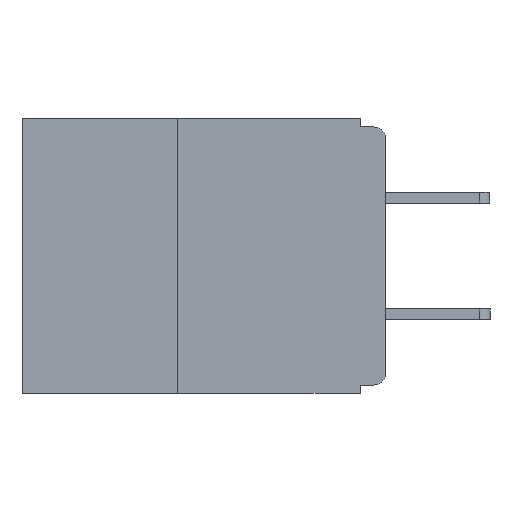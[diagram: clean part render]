
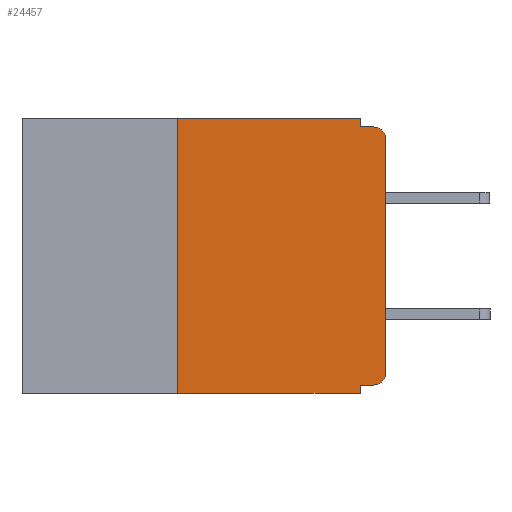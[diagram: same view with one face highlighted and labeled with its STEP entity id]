
A CAD part, left-side view. The second image highlights one B-rep face of the part: STEP entity #24457.
In plain terms, the highlighted planar face has unit normal (-1, 0, 0).
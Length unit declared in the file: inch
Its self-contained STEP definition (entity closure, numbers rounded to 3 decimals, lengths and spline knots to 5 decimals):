
#37 = VERTEX_POINT ( 'NONE', #17384 ) ;
#172 = LINE ( 'NONE', #26033, #16904 ) ;
#1233 = CIRCLE ( 'NONE', #4353, 0.015 ) ;
#1539 = LINE ( 'NONE', #8514, #12045 ) ;
#1706 = VERTEX_POINT ( 'NONE', #14903 ) ;
#2119 = VECTOR ( 'NONE', #4753, 39.37008 ) ;
#3079 = CARTESIAN_POINT ( 'NONE',  ( 0., 0.437, -0.33 ) ) ;
#3104 = DIRECTION ( 'NONE',  ( 0., -1., 0. ) ) ;
#3192 = EDGE_CURVE ( 'NONE', #7792, #24242, #1233, .T. ) ;
#3347 = CARTESIAN_POINT ( 'NONE',  ( 0., 0., -0.025 ) ) ;
#3579 = DIRECTION ( 'NONE',  ( 0., 0., -1. ) ) ;
#4067 = EDGE_CURVE ( 'NONE', #7661, #21349, #1539, .T. ) ;
#4260 = EDGE_LOOP ( 'NONE', ( #22981, #23502, #23554, #24234, #24512, #24639, #25040, #25345, #25352, #25629 ) ) ;
#4353 = AXIS2_PLACEMENT_3D ( 'NONE', #6481, #6469, #6438 ) ;
#4753 = DIRECTION ( 'NONE',  ( 0., 0., 1. ) ) ;
#4786 = CARTESIAN_POINT ( 'NONE',  ( 0., 0., 0. ) ) ;
#5506 = EDGE_CURVE ( 'NONE', #21349, #19329, #11683, .T. ) ;
#5776 = EDGE_CURVE ( 'NONE', #19329, #15866, #26083, .T. ) ;
#6105 = EDGE_CURVE ( 'NONE', #24242, #11061, #12623, .T. ) ;
#6438 = DIRECTION ( 'NONE',  ( 0., 0., -1. ) ) ;
#6469 = DIRECTION ( 'NONE',  ( -1., 0., 0. ) ) ;
#6481 = CARTESIAN_POINT ( 'NONE',  ( 0., 0.015, -0.305 ) ) ;
#7461 = PLANE ( 'NONE',  #7885 ) ;
#7475 = EDGE_CURVE ( 'NONE', #7792, #17585, #16513, .T. ) ;
#7661 = VERTEX_POINT ( 'NONE', #21266 ) ;
#7792 = VERTEX_POINT ( 'NONE', #18733 ) ;
#7885 = AXIS2_PLACEMENT_3D ( 'NONE', #9550, #11694, #26331 ) ;
#7938 = CARTESIAN_POINT ( 'NONE',  ( 0., 0.015, -0.025 ) ) ;
#8514 = CARTESIAN_POINT ( 'NONE',  ( 0., 0.25, -0.33 ) ) ;
#8648 = CARTESIAN_POINT ( 'NONE',  ( 0., 0., -0.305 ) ) ;
#8722 = CARTESIAN_POINT ( 'NONE',  ( 0., 0.031, -0.32 ) ) ;
#8989 = EDGE_CURVE ( 'NONE', #7661, #37, #23648, .T. ) ;
#9550 = CARTESIAN_POINT ( 'NONE',  ( 0., 0.437, 0. ) ) ;
#10058 = DIRECTION ( 'NONE',  ( 0., 0., -1. ) ) ;
#10143 = FACE_OUTER_BOUND ( 'NONE', #4260, .T. ) ;
#11061 = VERTEX_POINT ( 'NONE', #3347 ) ;
#11683 = LINE ( 'NONE', #17217, #16585 ) ;
#11694 = DIRECTION ( 'NONE',  ( 1., 0., 0. ) ) ;
#11939 = DIRECTION ( 'NONE',  ( 0., 0., -1. ) ) ;
#12045 = VECTOR ( 'NONE', #15084, 39.37008 ) ;
#12138 = CARTESIAN_POINT ( 'NONE',  ( 0., 0.031, 0. ) ) ;
#12623 = LINE ( 'NONE', #4786, #2119 ) ;
#13485 = DIRECTION ( 'NONE',  ( 0., -1., 0. ) ) ;
#13922 = EDGE_CURVE ( 'NONE', #17585, #37, #25687, .T. ) ;
#14903 = CARTESIAN_POINT ( 'NONE',  ( 0., 0.015, -0.01 ) ) ;
#15084 = DIRECTION ( 'NONE',  ( 0., 0., 1. ) ) ;
#15177 = VECTOR ( 'NONE', #3579, 39.37008 ) ;
#15866 = VERTEX_POINT ( 'NONE', #17449 ) ;
#16513 = LINE ( 'NONE', #23164, #26974 ) ;
#16585 = VECTOR ( 'NONE', #17040, 39.37008 ) ;
#16904 = VECTOR ( 'NONE', #13485, 39.37008 ) ;
#17040 = DIRECTION ( 'NONE',  ( 0., -1., 0. ) ) ;
#17217 = CARTESIAN_POINT ( 'NONE',  ( 0., 0.437, 0. ) ) ;
#17384 = CARTESIAN_POINT ( 'NONE',  ( 0., 0.031, -0.33 ) ) ;
#17449 = CARTESIAN_POINT ( 'NONE',  ( 0., 0.031, -0.01 ) ) ;
#17585 = VERTEX_POINT ( 'NONE', #8722 ) ;
#18733 = CARTESIAN_POINT ( 'NONE',  ( 0., 0.015, -0.32 ) ) ;
#18740 = VECTOR ( 'NONE', #3104, 39.37008 ) ;
#19329 = VERTEX_POINT ( 'NONE', #22797 ) ;
#20075 = AXIS2_PLACEMENT_3D ( 'NONE', #7938, #22610, #10058 ) ;
#20494 = VECTOR ( 'NONE', #11939, 39.37008 ) ;
#20536 = CARTESIAN_POINT ( 'NONE',  ( 0., 0.031, -0.33 ) ) ;
#20908 = EDGE_CURVE ( 'NONE', #11061, #1706, #23461, .T. ) ;
#21266 = CARTESIAN_POINT ( 'NONE',  ( 0., 0.25, -0.33 ) ) ;
#21291 = CARTESIAN_POINT ( 'NONE',  ( 0., 0.25, 0. ) ) ;
#21349 = VERTEX_POINT ( 'NONE', #21291 ) ;
#22104 = EDGE_CURVE ( 'NONE', #15866, #1706, #172, .T. ) ;
#22610 = DIRECTION ( 'NONE',  ( -1., 0., 0. ) ) ;
#22797 = CARTESIAN_POINT ( 'NONE',  ( 0., 0.031, 0. ) ) ;
#22981 = ORIENTED_EDGE ( 'NONE', *, *, #6105, .T. ) ;
#23103 = DIRECTION ( 'NONE',  ( 0., 1., 0. ) ) ;
#23164 = CARTESIAN_POINT ( 'NONE',  ( 0., 0., -0.32 ) ) ;
#23461 = CIRCLE ( 'NONE', #20075, 0.015 ) ;
#23502 = ORIENTED_EDGE ( 'NONE', *, *, #20908, .T. ) ;
#23554 = ORIENTED_EDGE ( 'NONE', *, *, #22104, .F. ) ;
#23648 = LINE ( 'NONE', #3079, #18740 ) ;
#24234 = ORIENTED_EDGE ( 'NONE', *, *, #5776, .F. ) ;
#24242 = VERTEX_POINT ( 'NONE', #8648 ) ;
#24457 = ADVANCED_FACE ( 'NONE', ( #10143 ), #7461, .F. ) ;
#24512 = ORIENTED_EDGE ( 'NONE', *, *, #5506, .F. ) ;
#24639 = ORIENTED_EDGE ( 'NONE', *, *, #4067, .F. ) ;
#25040 = ORIENTED_EDGE ( 'NONE', *, *, #8989, .T. ) ;
#25345 = ORIENTED_EDGE ( 'NONE', *, *, #13922, .F. ) ;
#25352 = ORIENTED_EDGE ( 'NONE', *, *, #7475, .F. ) ;
#25629 = ORIENTED_EDGE ( 'NONE', *, *, #3192, .T. ) ;
#25687 = LINE ( 'NONE', #20536, #15177 ) ;
#26033 = CARTESIAN_POINT ( 'NONE',  ( 0., 0., -0.01 ) ) ;
#26083 = LINE ( 'NONE', #12138, #20494 ) ;
#26331 = DIRECTION ( 'NONE',  ( 0., 0., -1. ) ) ;
#26974 = VECTOR ( 'NONE', #23103, 39.37008 ) ;
